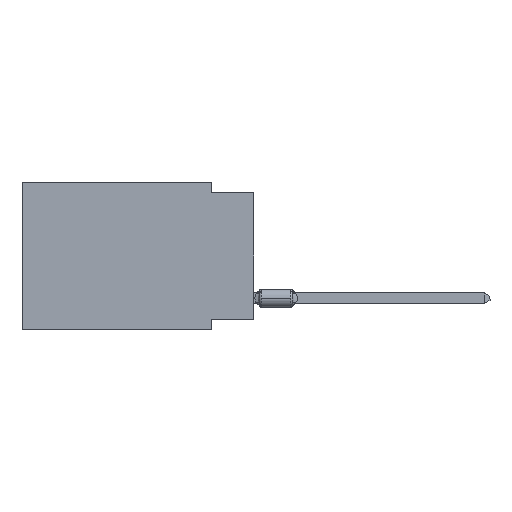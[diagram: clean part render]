
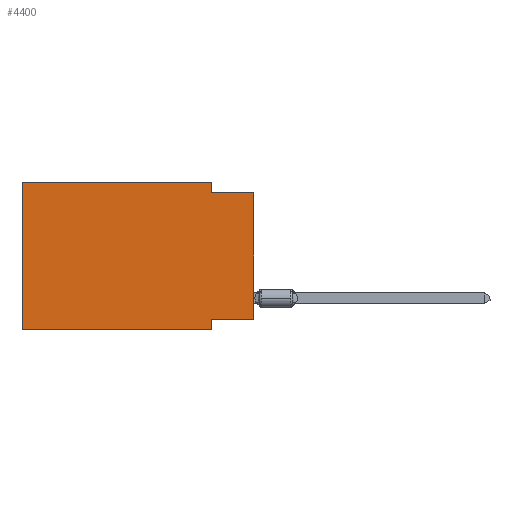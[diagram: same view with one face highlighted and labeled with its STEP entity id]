
A CAD part, left-side view. The second image highlights one B-rep face of the part: STEP entity #4400.
In plain terms, the highlighted planar face has unit normal (-1, 0, 0).
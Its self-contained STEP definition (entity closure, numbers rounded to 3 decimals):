
#30 = EDGE_CURVE ( 'NONE', #15648, #24213, #14689, .T. ) ;
#83 = LINE ( 'NONE', #22665, #2910 ) ;
#394 = CARTESIAN_POINT ( 'NONE',  ( 0., 0., 0. ) ) ;
#470 = EDGE_CURVE ( 'NONE', #12528, #6971, #21758, .T. ) ;
#1585 = CARTESIAN_POINT ( 'NONE',  ( 0., 0., -8.255 ) ) ;
#2133 = ORIENTED_EDGE ( 'NONE', *, *, #4774, .T. ) ;
#2864 = CARTESIAN_POINT ( 'NONE',  ( 0., 2.54, 0. ) ) ;
#2910 = VECTOR ( 'NONE', #11224, 1000. ) ;
#3526 = ORIENTED_EDGE ( 'NONE', *, *, #17690, .F. ) ;
#4061 = DIRECTION ( 'NONE',  ( 0., 0., 1. ) ) ;
#4102 = CARTESIAN_POINT ( 'NONE',  ( 0., 13.97, 0. ) ) ;
#4138 = DIRECTION ( 'NONE',  ( 0., -1., 0. ) ) ;
#4400 = ADVANCED_FACE ( 'NONE', ( #15254 ), #15006, .F. ) ;
#4506 = VERTEX_POINT ( 'NONE', #6937 ) ;
#4774 = EDGE_CURVE ( 'NONE', #15648, #10631, #6321, .T. ) ;
#5136 = LINE ( 'NONE', #1585, #22696 ) ;
#5550 = EDGE_CURVE ( 'NONE', #6971, #7820, #13446, .T. ) ;
#5684 = DIRECTION ( 'NONE',  ( 0., 0., -1. ) ) ;
#5798 = ORIENTED_EDGE ( 'NONE', *, *, #30, .F. ) ;
#6141 = ORIENTED_EDGE ( 'NONE', *, *, #470, .F. ) ;
#6321 = LINE ( 'NONE', #6551, #12996 ) ;
#6551 = CARTESIAN_POINT ( 'NONE',  ( 0., 13.97, -8.89 ) ) ;
#6937 = CARTESIAN_POINT ( 'NONE',  ( 0., 0., -8.255 ) ) ;
#6953 = DIRECTION ( 'NONE',  ( 0., 1., 0. ) ) ;
#6971 = VERTEX_POINT ( 'NONE', #11352 ) ;
#7001 = EDGE_CURVE ( 'NONE', #14899, #10631, #83, .T. ) ;
#7288 = VECTOR ( 'NONE', #4061, 1000. ) ;
#7479 = ORIENTED_EDGE ( 'NONE', *, *, #18562, .T. ) ;
#7820 = VERTEX_POINT ( 'NONE', #11995 ) ;
#7821 = CARTESIAN_POINT ( 'NONE',  ( 0., 13.97, -8.89 ) ) ;
#8273 = CARTESIAN_POINT ( 'NONE',  ( 0., 2.54, -8.89 ) ) ;
#8470 = VECTOR ( 'NONE', #12845, 1000. ) ;
#8787 = EDGE_LOOP ( 'NONE', ( #7479, #16166, #6141, #3526, #5798, #2133, #15994, #9988 ) ) ;
#9722 = CARTESIAN_POINT ( 'NONE',  ( 0., 13.97, 0. ) ) ;
#9988 = ORIENTED_EDGE ( 'NONE', *, *, #23429, .F. ) ;
#10631 = VERTEX_POINT ( 'NONE', #8273 ) ;
#11224 = DIRECTION ( 'NONE',  ( 0., 0., -1. ) ) ;
#11352 = CARTESIAN_POINT ( 'NONE',  ( 0., 2.54, -0.635 ) ) ;
#11413 = AXIS2_PLACEMENT_3D ( 'NONE', #17217, #22516, #5684 ) ;
#11995 = CARTESIAN_POINT ( 'NONE',  ( 0., 0., -0.635 ) ) ;
#12522 = CARTESIAN_POINT ( 'NONE',  ( 0., 2.54, -8.255 ) ) ;
#12528 = VERTEX_POINT ( 'NONE', #18738 ) ;
#12845 = DIRECTION ( 'NONE',  ( 0., 0., 1. ) ) ;
#12996 = VECTOR ( 'NONE', #13799, 1000. ) ;
#13446 = LINE ( 'NONE', #21220, #23605 ) ;
#13799 = DIRECTION ( 'NONE',  ( 0., -1., 0. ) ) ;
#14689 = LINE ( 'NONE', #22189, #8470 ) ;
#14899 = VERTEX_POINT ( 'NONE', #12522 ) ;
#15006 = PLANE ( 'NONE',  #11413 ) ;
#15254 = FACE_OUTER_BOUND ( 'NONE', #8787, .T. ) ;
#15648 = VERTEX_POINT ( 'NONE', #7821 ) ;
#15994 = ORIENTED_EDGE ( 'NONE', *, *, #7001, .F. ) ;
#16166 = ORIENTED_EDGE ( 'NONE', *, *, #5550, .F. ) ;
#17179 = LINE ( 'NONE', #394, #7288 ) ;
#17217 = CARTESIAN_POINT ( 'NONE',  ( 0., 13.97, 0. ) ) ;
#17690 = EDGE_CURVE ( 'NONE', #24213, #12528, #22893, .T. ) ;
#18562 = EDGE_CURVE ( 'NONE', #4506, #7820, #17179, .T. ) ;
#18738 = CARTESIAN_POINT ( 'NONE',  ( 0., 2.54, 0. ) ) ;
#19074 = DIRECTION ( 'NONE',  ( 0., -1., 0. ) ) ;
#19445 = VECTOR ( 'NONE', #19074, 1000. ) ;
#19896 = VECTOR ( 'NONE', #21297, 1000. ) ;
#21220 = CARTESIAN_POINT ( 'NONE',  ( 0., 0., -0.635 ) ) ;
#21297 = DIRECTION ( 'NONE',  ( 0., 0., -1. ) ) ;
#21758 = LINE ( 'NONE', #2864, #19896 ) ;
#22189 = CARTESIAN_POINT ( 'NONE',  ( 0., 13.97, 0. ) ) ;
#22516 = DIRECTION ( 'NONE',  ( 1., 0., 0. ) ) ;
#22665 = CARTESIAN_POINT ( 'NONE',  ( 0., 2.54, -8.89 ) ) ;
#22696 = VECTOR ( 'NONE', #6953, 1000. ) ;
#22893 = LINE ( 'NONE', #4102, #19445 ) ;
#23429 = EDGE_CURVE ( 'NONE', #4506, #14899, #5136, .T. ) ;
#23605 = VECTOR ( 'NONE', #4138, 1000. ) ;
#24213 = VERTEX_POINT ( 'NONE', #9722 ) ;
